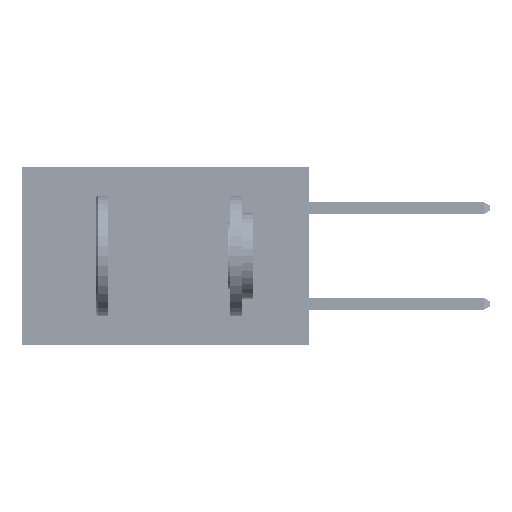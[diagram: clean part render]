
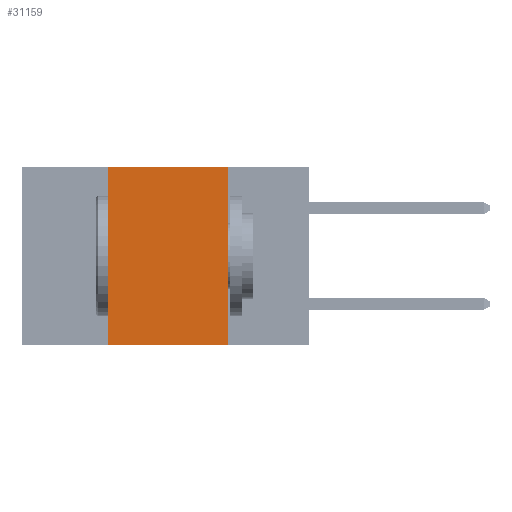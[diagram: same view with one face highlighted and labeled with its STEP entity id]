
A CAD part, left-side view. The second image highlights one B-rep face of the part: STEP entity #31159.
In plain terms, the highlighted planar face has unit normal (-1, 0, 0).
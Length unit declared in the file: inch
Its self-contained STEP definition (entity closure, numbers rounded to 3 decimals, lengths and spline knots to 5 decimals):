
#1410 = AXIS2_PLACEMENT_3D ( 'NONE', #40638, #1988, #44221 ) ;
#1988 = DIRECTION ( 'NONE',  ( 1., 0., 0. ) ) ;
#3163 = VERTEX_POINT ( 'NONE', #15599 ) ;
#4035 = CARTESIAN_POINT ( 'NONE',  ( 0., 0.42, 0. ) ) ;
#6620 = FACE_OUTER_BOUND ( 'NONE', #33125, .T. ) ;
#7874 = DIRECTION ( 'NONE',  ( 0., 0., -1. ) ) ;
#8249 = LINE ( 'NONE', #11743, #43272 ) ;
#8951 = ORIENTED_EDGE ( 'NONE', *, *, #41632, .T. ) ;
#11743 = CARTESIAN_POINT ( 'NONE',  ( 0., 0.6, -0.37 ) ) ;
#11890 = CARTESIAN_POINT ( 'NONE',  ( 0., 0.17, 0. ) ) ;
#14890 = CARTESIAN_POINT ( 'NONE',  ( 0., 0.6, 0. ) ) ;
#14977 = LINE ( 'NONE', #23040, #37352 ) ;
#15599 = CARTESIAN_POINT ( 'NONE',  ( 0., 0.17, -0.37 ) ) ;
#15796 = CARTESIAN_POINT ( 'NONE',  ( 0., 0.17, 0. ) ) ;
#19671 = DIRECTION ( 'NONE',  ( 0., -1., 0. ) ) ;
#21603 = VECTOR ( 'NONE', #7874, 39.37008 ) ;
#21885 = EDGE_CURVE ( 'NONE', #36443, #3163, #43990, .T. ) ;
#22028 = LINE ( 'NONE', #14890, #30512 ) ;
#22490 = DIRECTION ( 'NONE',  ( 0., -1., 0. ) ) ;
#23040 = CARTESIAN_POINT ( 'NONE',  ( 0., 0.42, 0. ) ) ;
#24896 = CARTESIAN_POINT ( 'NONE',  ( 0., 0.42, -0.37 ) ) ;
#27375 = EDGE_CURVE ( 'NONE', #39166, #47275, #14977, .T. ) ;
#27643 = ORIENTED_EDGE ( 'NONE', *, *, #27375, .F. ) ;
#30512 = VECTOR ( 'NONE', #22490, 39.37008 ) ;
#31159 = ADVANCED_FACE ( 'NONE', ( #6620 ), #36643, .F. ) ;
#33125 = EDGE_LOOP ( 'NONE', ( #49948, #42075, #27643, #8951 ) ) ;
#36443 = VERTEX_POINT ( 'NONE', #11890 ) ;
#36643 = PLANE ( 'NONE',  #1410 ) ;
#37352 = VECTOR ( 'NONE', #38429, 39.37008 ) ;
#38429 = DIRECTION ( 'NONE',  ( 0., 0., 1. ) ) ;
#39166 = VERTEX_POINT ( 'NONE', #24896 ) ;
#40638 = CARTESIAN_POINT ( 'NONE',  ( 0., 0.6, 0. ) ) ;
#41632 = EDGE_CURVE ( 'NONE', #39166, #3163, #8249, .T. ) ;
#42075 = ORIENTED_EDGE ( 'NONE', *, *, #44024, .F. ) ;
#43272 = VECTOR ( 'NONE', #19671, 39.37008 ) ;
#43990 = LINE ( 'NONE', #15796, #21603 ) ;
#44024 = EDGE_CURVE ( 'NONE', #47275, #36443, #22028, .T. ) ;
#44221 = DIRECTION ( 'NONE',  ( 0., 0., -1. ) ) ;
#47275 = VERTEX_POINT ( 'NONE', #4035 ) ;
#49948 = ORIENTED_EDGE ( 'NONE', *, *, #21885, .F. ) ;
